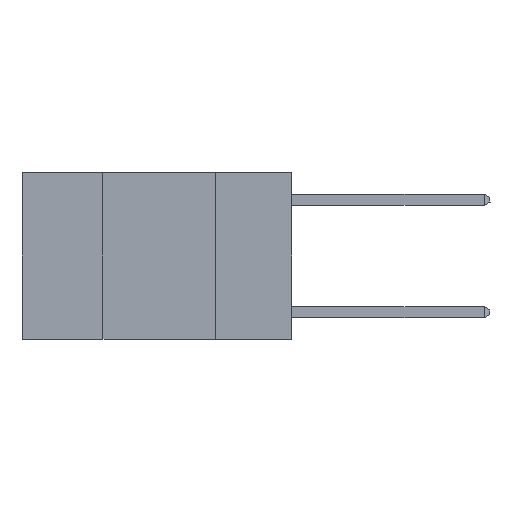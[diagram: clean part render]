
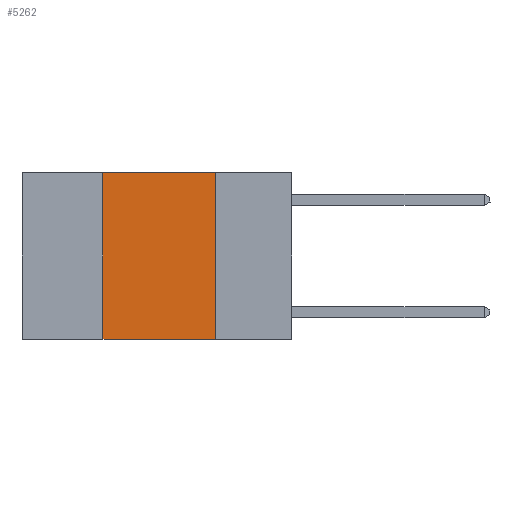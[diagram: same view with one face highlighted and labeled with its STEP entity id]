
A CAD part, left-side view. The second image highlights one B-rep face of the part: STEP entity #5262.
In plain terms, the highlighted planar face has unit normal (-1, 0, 0).
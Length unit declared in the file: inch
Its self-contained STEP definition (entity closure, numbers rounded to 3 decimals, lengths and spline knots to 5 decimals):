
#163 = VERTEX_POINT ( 'NONE', #616 ) ;
#616 = CARTESIAN_POINT ( 'NONE',  ( 0., 0.42, -0.37 ) ) ;
#763 = CARTESIAN_POINT ( 'NONE',  ( 0., 0.17, 0. ) ) ;
#783 = DIRECTION ( 'NONE',  ( 0., 0., -1. ) ) ;
#1807 = EDGE_CURVE ( 'NONE', #10078, #6614, #6755, .T. ) ;
#2429 = PLANE ( 'NONE',  #14611 ) ;
#2776 = LINE ( 'NONE', #8046, #9444 ) ;
#3419 = VECTOR ( 'NONE', #6922, 39.37008 ) ;
#3483 = DIRECTION ( 'NONE',  ( 0., 0., -1. ) ) ;
#3586 = FACE_OUTER_BOUND ( 'NONE', #10023, .T. ) ;
#4791 = DIRECTION ( 'NONE',  ( 1., 0., 0. ) ) ;
#5262 = ADVANCED_FACE ( 'NONE', ( #3586 ), #2429, .F. ) ;
#6134 = VERTEX_POINT ( 'NONE', #10220 ) ;
#6614 = VERTEX_POINT ( 'NONE', #16886 ) ;
#6755 = LINE ( 'NONE', #6838, #3419 ) ;
#6838 = CARTESIAN_POINT ( 'NONE',  ( 0., 0.6, 0. ) ) ;
#6922 = DIRECTION ( 'NONE',  ( 0., -1., 0. ) ) ;
#7504 = VECTOR ( 'NONE', #15394, 39.37008 ) ;
#7956 = DIRECTION ( 'NONE',  ( 0., -1., 0. ) ) ;
#8046 = CARTESIAN_POINT ( 'NONE',  ( 0., 0.6, -0.37 ) ) ;
#8858 = CARTESIAN_POINT ( 'NONE',  ( 0., 0.6, 0. ) ) ;
#9444 = VECTOR ( 'NONE', #7956, 39.37008 ) ;
#10023 = EDGE_LOOP ( 'NONE', ( #15391, #11179, #16916, #10650 ) ) ;
#10078 = VERTEX_POINT ( 'NONE', #12034 ) ;
#10220 = CARTESIAN_POINT ( 'NONE',  ( 0., 0.17, -0.37 ) ) ;
#10650 = ORIENTED_EDGE ( 'NONE', *, *, #14506, .T. ) ;
#11179 = ORIENTED_EDGE ( 'NONE', *, *, #1807, .F. ) ;
#11249 = LINE ( 'NONE', #763, #16353 ) ;
#12034 = CARTESIAN_POINT ( 'NONE',  ( 0., 0.42, 0. ) ) ;
#13501 = EDGE_CURVE ( 'NONE', #6614, #6134, #11249, .T. ) ;
#14506 = EDGE_CURVE ( 'NONE', #163, #6134, #2776, .T. ) ;
#14611 = AXIS2_PLACEMENT_3D ( 'NONE', #8858, #4791, #783 ) ;
#15391 = ORIENTED_EDGE ( 'NONE', *, *, #13501, .F. ) ;
#15394 = DIRECTION ( 'NONE',  ( 0., 0., 1. ) ) ;
#16353 = VECTOR ( 'NONE', #3483, 39.37008 ) ;
#16483 = EDGE_CURVE ( 'NONE', #163, #10078, #16762, .T. ) ;
#16762 = LINE ( 'NONE', #16845, #7504 ) ;
#16845 = CARTESIAN_POINT ( 'NONE',  ( 0., 0.42, 0. ) ) ;
#16886 = CARTESIAN_POINT ( 'NONE',  ( 0., 0.17, 0. ) ) ;
#16916 = ORIENTED_EDGE ( 'NONE', *, *, #16483, .F. ) ;
